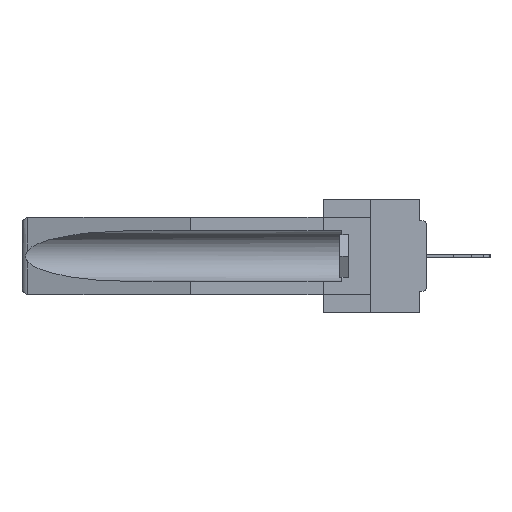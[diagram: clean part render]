
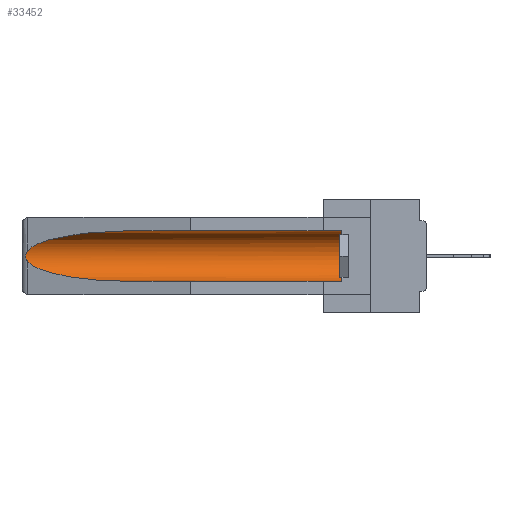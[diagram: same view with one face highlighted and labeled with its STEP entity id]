
A CAD part, left-side view. The second image highlights one B-rep face of the part: STEP entity #33452.
In plain terms, the highlighted cylindrical face has radius 2.857 mm (diameter 5.715 mm), a partial arc.
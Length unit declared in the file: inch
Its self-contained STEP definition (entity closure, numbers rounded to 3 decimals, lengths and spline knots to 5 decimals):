
#40 = EDGE_CURVE ( 'NONE', #4344, #9771, #10853, .T. ) ;
#86 = CARTESIAN_POINT ( 'NONE',  ( 0.26537, 1.52718, -0.14972 ) ) ;
#422 = ORIENTED_EDGE ( 'NONE', *, *, #12120, .F. ) ;
#1249 = CARTESIAN_POINT ( 'NONE',  ( 0.155, 1.07973, -0.284 ) ) ;
#1811 = VERTEX_POINT ( 'NONE', #7892 ) ;
#1993 = EDGE_CURVE ( 'NONE', #10792, #1811, #26372, .T. ) ;
#2343 = CIRCLE ( 'NONE', #27461, 0.1125 ) ;
#2756 = DIRECTION ( 'NONE',  ( 0., 0., 1. ) ) ;
#2757 = CARTESIAN_POINT ( 'NONE',  ( 0.26537, 1.52718, -0.14972 ) ) ;
#3111 = ORIENTED_EDGE ( 'NONE', *, *, #40, .T. ) ;
#3447 = DIRECTION ( 'NONE',  ( 0., 1., 0. ) ) ;
#3717 = AXIS2_PLACEMENT_3D ( 'NONE', #20275, #4564, #14858 ) ;
#3879 = CARTESIAN_POINT ( 'NONE',  ( 0.26537, 1.52718, -0.19328 ) ) ;
#4297 = CARTESIAN_POINT ( 'NONE',  ( 0.26537, 1.52718, -0.14972 ) ) ;
#4344 = VERTEX_POINT ( 'NONE', #19676 ) ;
#4539 = CARTESIAN_POINT ( 'NONE',  ( 0.155, 0.126, -0.284 ) ) ;
#4564 = DIRECTION ( 'NONE',  ( 0., 1., 0. ) ) ;
#5327 = CARTESIAN_POINT ( 'NONE',  ( 0.26597, 1.52961, -0.15275 ) ) ;
#6493 = EDGE_CURVE ( 'NONE', #9771, #24086, #18289, .T. ) ;
#6665 = CARTESIAN_POINT ( 'NONE',  ( 0.21114, 1.30732, -0.284 ) ) ;
#7892 = CARTESIAN_POINT ( 'NONE',  ( 0.155, 1.07973, -0.284 ) ) ;
#8318 = ORIENTED_EDGE ( 'NONE', *, *, #13924, .T. ) ;
#8721 = VECTOR ( 'NONE', #11032, 39.37008 ) ;
#8940 = EDGE_LOOP ( 'NONE', ( #13914, #8318, #27056, #422, #22765, #3111 ) ) ;
#9536 = CARTESIAN_POINT ( 'NONE',  ( 0.155, 1.07973, -0.059 ) ) ;
#9771 = VERTEX_POINT ( 'NONE', #22254 ) ;
#10379 = VERTEX_POINT ( 'NONE', #4539 ) ;
#10792 = VERTEX_POINT ( 'NONE', #14791 ) ;
#10853 = LINE ( 'NONE', #13805, #8721 ) ;
#11032 = DIRECTION ( 'NONE',  ( 0., 1., 0. ) ) ;
#11276 = VECTOR ( 'NONE', #3447, 39.37008 ) ;
#11823 = LINE ( 'NONE', #17068, #11276 ) ;
#11902 = EDGE_CURVE ( 'NONE', #10379, #4344, #2343, .T. ) ;
#12120 = EDGE_CURVE ( 'NONE', #10379, #1811, #11823, .T. ) ;
#13805 = CARTESIAN_POINT ( 'NONE',  ( 0.155, -0.30754, -0.059 ) ) ;
#13914 = ORIENTED_EDGE ( 'NONE', *, *, #6493, .T. ) ;
#13924 = EDGE_CURVE ( 'NONE', #24086, #10792, #19645, .T. ) ;
#14791 = CARTESIAN_POINT ( 'NONE',  ( 0.26537, 1.52718, -0.19328 ) ) ;
#14858 = DIRECTION ( 'NONE',  ( 0., 0., 1. ) ) ;
#17068 = CARTESIAN_POINT ( 'NONE',  ( 0.155, -0.30754, -0.284 ) ) ;
#17549 = CARTESIAN_POINT ( 'NONE',  ( 0.25451, 1.48313, -0.09465 ) ) ;
#17593 = CARTESIAN_POINT ( 'NONE',  ( 0.155, 0.126, -0.1715 ) ) ;
#18289 =( BOUNDED_CURVE ( )  B_SPLINE_CURVE ( 3, ( #9536, #28249, #17549, #4297 ),
 .UNSPECIFIED., .F., .F. ) 
 B_SPLINE_CURVE_WITH_KNOTS ( ( 4, 4 ),
 ( 4.71239, 6.08839 ),
 .UNSPECIFIED. ) 
 CURVE ( )  GEOMETRIC_REPRESENTATION_ITEM ( )  RATIONAL_B_SPLINE_CURVE ( ( 1., 0.848, 0.848, 1. ) ) 
 REPRESENTATION_ITEM ( '' )  );
#18940 = CARTESIAN_POINT ( 'NONE',  ( 0.2675, 1.53308, -0.16763 ) ) ;
#19645 = B_SPLINE_CURVE_WITH_KNOTS ( 'NONE', 3,
 ( #86, #5327, #24190, #24018, #18940, #32091, #29261, #26481, #26838, #32436 ),
 .UNSPECIFIED., .F., .F.,
 ( 4, 2, 2, 2, 4 ),
 ( 0., 0.00029, 0.00058, 0.00087, 0.00117 ),
 .UNSPECIFIED. ) ;
#19676 = CARTESIAN_POINT ( 'NONE',  ( 0.155, 0.126, -0.059 ) ) ;
#20275 = CARTESIAN_POINT ( 'NONE',  ( 0.155, -0.30754, -0.1715 ) ) ;
#22254 = CARTESIAN_POINT ( 'NONE',  ( 0.155, 1.07973, -0.059 ) ) ;
#22765 = ORIENTED_EDGE ( 'NONE', *, *, #11902, .T. ) ;
#24018 = CARTESIAN_POINT ( 'NONE',  ( 0.2673, 1.5327, -0.16383 ) ) ;
#24086 = VERTEX_POINT ( 'NONE', #2757 ) ;
#24190 = CARTESIAN_POINT ( 'NONE',  ( 0.26654, 1.53092, -0.15636 ) ) ;
#26372 =( BOUNDED_CURVE ( )  B_SPLINE_CURVE ( 3, ( #3879, #30789, #6665, #1249 ),
 .UNSPECIFIED., .F., .F. ) 
 B_SPLINE_CURVE_WITH_KNOTS ( ( 4, 4 ),
 ( 0.1948, 1.5708 ),
 .UNSPECIFIED. ) 
 CURVE ( )  GEOMETRIC_REPRESENTATION_ITEM ( )  RATIONAL_B_SPLINE_CURVE ( ( 1., 0.848, 0.848, 1. ) ) 
 REPRESENTATION_ITEM ( '' )  );
#26481 = CARTESIAN_POINT ( 'NONE',  ( 0.26655, 1.53094, -0.18657 ) ) ;
#26838 = CARTESIAN_POINT ( 'NONE',  ( 0.26597, 1.5296, -0.19026 ) ) ;
#27056 = ORIENTED_EDGE ( 'NONE', *, *, #1993, .T. ) ;
#27461 = AXIS2_PLACEMENT_3D ( 'NONE', #17593, #33696, #2756 ) ;
#28181 = FACE_OUTER_BOUND ( 'NONE', #8940, .T. ) ;
#28249 = CARTESIAN_POINT ( 'NONE',  ( 0.21114, 1.30732, -0.059 ) ) ;
#29261 = CARTESIAN_POINT ( 'NONE',  ( 0.2673, 1.53269, -0.17917 ) ) ;
#30789 = CARTESIAN_POINT ( 'NONE',  ( 0.25451, 1.48313, -0.24835 ) ) ;
#32091 = CARTESIAN_POINT ( 'NONE',  ( 0.2675, 1.53308, -0.17534 ) ) ;
#32436 = CARTESIAN_POINT ( 'NONE',  ( 0.26537, 1.52718, -0.19328 ) ) ;
#33435 = CYLINDRICAL_SURFACE ( 'NONE', #3717, 0.1125 ) ;
#33452 = ADVANCED_FACE ( 'NONE', ( #28181 ), #33435, .F. ) ;
#33696 = DIRECTION ( 'NONE',  ( 0., -1., 0. ) ) ;
